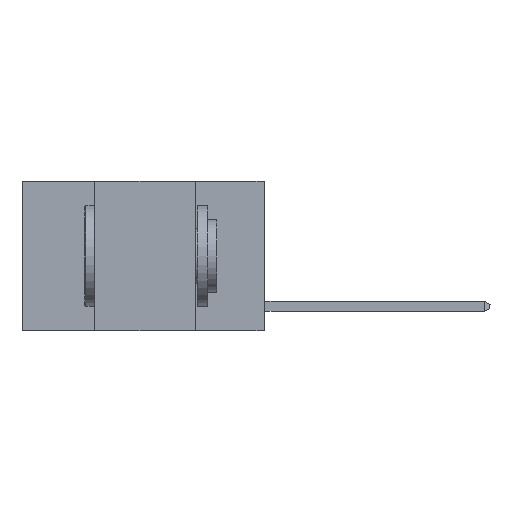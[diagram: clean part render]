
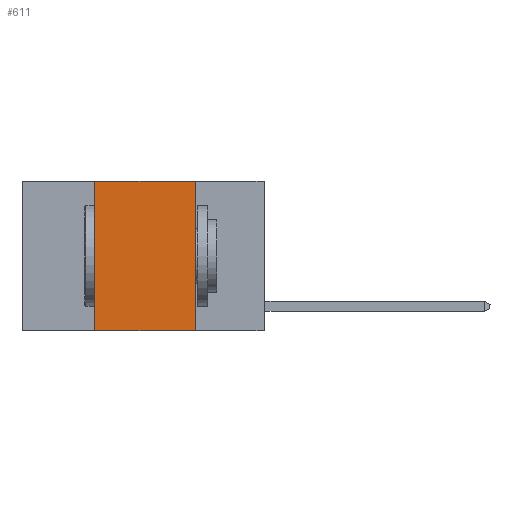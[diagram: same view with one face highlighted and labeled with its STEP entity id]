
A CAD part, left-side view. The second image highlights one B-rep face of the part: STEP entity #611.
In plain terms, the highlighted planar face has unit normal (-1, 0, 0).
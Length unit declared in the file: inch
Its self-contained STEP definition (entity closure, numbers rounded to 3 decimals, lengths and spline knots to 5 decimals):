
#611 = ADVANCED_FACE ( 'NONE', ( #20019 ), #17717, .F. ) ;
#628 = LINE ( 'NONE', #21238, #10535 ) ;
#1569 = VERTEX_POINT ( 'NONE', #7777 ) ;
#1718 = CARTESIAN_POINT ( 'NONE',  ( 0., 0.42, 0. ) ) ;
#1984 = EDGE_CURVE ( 'NONE', #19003, #1569, #15313, .T. ) ;
#4198 = ORIENTED_EDGE ( 'NONE', *, *, #22784, .F. ) ;
#7288 = DIRECTION ( 'NONE',  ( 0., 0., 1. ) ) ;
#7617 = CARTESIAN_POINT ( 'NONE',  ( 0., 0.6, -0.37 ) ) ;
#7777 = CARTESIAN_POINT ( 'NONE',  ( 0., 0.17, -0.37 ) ) ;
#8870 = DIRECTION ( 'NONE',  ( 0., -1., 0. ) ) ;
#9528 = EDGE_CURVE ( 'NONE', #19744, #19997, #628, .T. ) ;
#9893 = ORIENTED_EDGE ( 'NONE', *, *, #1984, .T. ) ;
#10072 = ORIENTED_EDGE ( 'NONE', *, *, #25096, .F. ) ;
#10515 = CARTESIAN_POINT ( 'NONE',  ( 0., 0.17, 0. ) ) ;
#10535 = VECTOR ( 'NONE', #8870, 39.37008 ) ;
#10668 = EDGE_LOOP ( 'NONE', ( #10072, #25786, #4198, #9893 ) ) ;
#10810 = DIRECTION ( 'NONE',  ( 0., 0., -1. ) ) ;
#13301 = LINE ( 'NONE', #17767, #22177 ) ;
#15313 = LINE ( 'NONE', #7617, #20054 ) ;
#15387 = VECTOR ( 'NONE', #10810, 39.37008 ) ;
#15664 = DIRECTION ( 'NONE',  ( 0., 0., -1. ) ) ;
#15832 = DIRECTION ( 'NONE',  ( 1., 0., 0. ) ) ;
#17717 = PLANE ( 'NONE',  #25773 ) ;
#17742 = DIRECTION ( 'NONE',  ( 0., -1., 0. ) ) ;
#17767 = CARTESIAN_POINT ( 'NONE',  ( 0., 0.42, 0. ) ) ;
#17787 = CARTESIAN_POINT ( 'NONE',  ( 0., 0.42, -0.37 ) ) ;
#19003 = VERTEX_POINT ( 'NONE', #17787 ) ;
#19744 = VERTEX_POINT ( 'NONE', #1718 ) ;
#19997 = VERTEX_POINT ( 'NONE', #10515 ) ;
#20019 = FACE_OUTER_BOUND ( 'NONE', #10668, .T. ) ;
#20054 = VECTOR ( 'NONE', #17742, 39.37008 ) ;
#21238 = CARTESIAN_POINT ( 'NONE',  ( 0., 0.6, 0. ) ) ;
#22177 = VECTOR ( 'NONE', #7288, 39.37008 ) ;
#22665 = LINE ( 'NONE', #26260, #15387 ) ;
#22784 = EDGE_CURVE ( 'NONE', #19003, #19744, #13301, .T. ) ;
#25096 = EDGE_CURVE ( 'NONE', #19997, #1569, #22665, .T. ) ;
#25685 = CARTESIAN_POINT ( 'NONE',  ( 0., 0.6, 0. ) ) ;
#25773 = AXIS2_PLACEMENT_3D ( 'NONE', #25685, #15832, #15664 ) ;
#25786 = ORIENTED_EDGE ( 'NONE', *, *, #9528, .F. ) ;
#26260 = CARTESIAN_POINT ( 'NONE',  ( 0., 0.17, 0. ) ) ;
